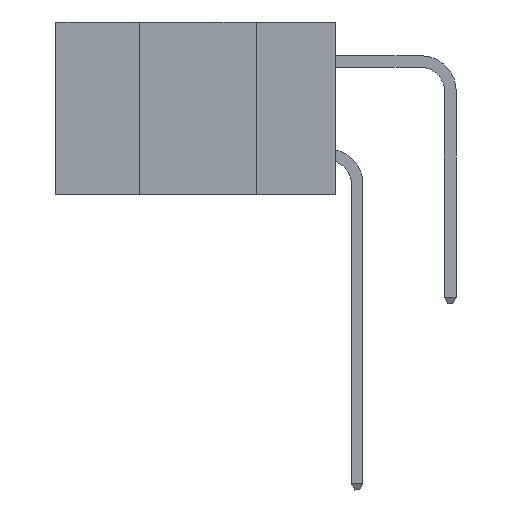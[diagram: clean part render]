
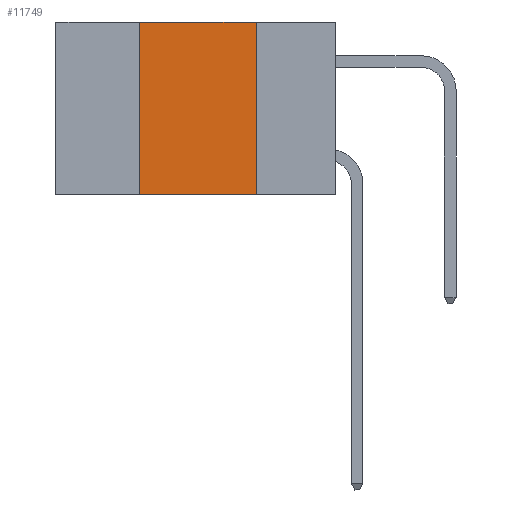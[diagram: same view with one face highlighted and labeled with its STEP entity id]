
A CAD part, left-side view. The second image highlights one B-rep face of the part: STEP entity #11749.
In plain terms, the highlighted planar face has unit normal (-1, 0, 0).
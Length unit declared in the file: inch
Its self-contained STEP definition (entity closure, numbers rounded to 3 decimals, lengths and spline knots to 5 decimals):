
#2803 = EDGE_CURVE ( 'NONE', #36819, #23230, #16107, .T. ) ;
#5247 = VERTEX_POINT ( 'NONE', #18322 ) ;
#5540 = VECTOR ( 'NONE', #14625, 39.37008 ) ;
#7446 = EDGE_CURVE ( 'NONE', #5247, #23230, #14202, .T. ) ;
#7920 = DIRECTION ( 'NONE',  ( 0., -1., 0. ) ) ;
#8594 = LINE ( 'NONE', #22272, #41772 ) ;
#9420 = FACE_OUTER_BOUND ( 'NONE', #20045, .T. ) ;
#9464 = CARTESIAN_POINT ( 'NONE',  ( 0., 0.17, 0. ) ) ;
#11749 = ADVANCED_FACE ( 'NONE', ( #9420 ), #23096, .F. ) ;
#12534 = ORIENTED_EDGE ( 'NONE', *, *, #7446, .T. ) ;
#14202 = LINE ( 'NONE', #25184, #18801 ) ;
#14625 = DIRECTION ( 'NONE',  ( 0., -1., 0. ) ) ;
#15187 = AXIS2_PLACEMENT_3D ( 'NONE', #33654, #39904, #30510 ) ;
#16107 = LINE ( 'NONE', #33630, #39212 ) ;
#16855 = CARTESIAN_POINT ( 'NONE',  ( 0., 0.42, 0. ) ) ;
#18322 = CARTESIAN_POINT ( 'NONE',  ( 0., 0.42, -0.37 ) ) ;
#18600 = CARTESIAN_POINT ( 'NONE',  ( 0., 0.17, -0.37 ) ) ;
#18801 = VECTOR ( 'NONE', #7920, 39.37008 ) ;
#20045 = EDGE_LOOP ( 'NONE', ( #38130, #43483, #41602, #12534 ) ) ;
#22272 = CARTESIAN_POINT ( 'NONE',  ( 0., 0.42, 0. ) ) ;
#23096 = PLANE ( 'NONE',  #15187 ) ;
#23230 = VERTEX_POINT ( 'NONE', #18600 ) ;
#25184 = CARTESIAN_POINT ( 'NONE',  ( 0., 0.6, -0.37 ) ) ;
#25275 = EDGE_CURVE ( 'NONE', #32839, #36819, #41535, .T. ) ;
#29374 = DIRECTION ( 'NONE',  ( 0., 0., -1. ) ) ;
#30510 = DIRECTION ( 'NONE',  ( 0., 0., -1. ) ) ;
#32839 = VERTEX_POINT ( 'NONE', #16855 ) ;
#33630 = CARTESIAN_POINT ( 'NONE',  ( 0., 0.17, 0. ) ) ;
#33654 = CARTESIAN_POINT ( 'NONE',  ( 0., 0.6, 0. ) ) ;
#35049 = CARTESIAN_POINT ( 'NONE',  ( 0., 0.6, 0. ) ) ;
#35085 = DIRECTION ( 'NONE',  ( 0., 0., 1. ) ) ;
#35418 = EDGE_CURVE ( 'NONE', #5247, #32839, #8594, .T. ) ;
#36819 = VERTEX_POINT ( 'NONE', #9464 ) ;
#38130 = ORIENTED_EDGE ( 'NONE', *, *, #2803, .F. ) ;
#39212 = VECTOR ( 'NONE', #29374, 39.37008 ) ;
#39904 = DIRECTION ( 'NONE',  ( 1., 0., 0. ) ) ;
#41535 = LINE ( 'NONE', #35049, #5540 ) ;
#41602 = ORIENTED_EDGE ( 'NONE', *, *, #35418, .F. ) ;
#41772 = VECTOR ( 'NONE', #35085, 39.37008 ) ;
#43483 = ORIENTED_EDGE ( 'NONE', *, *, #25275, .F. ) ;
